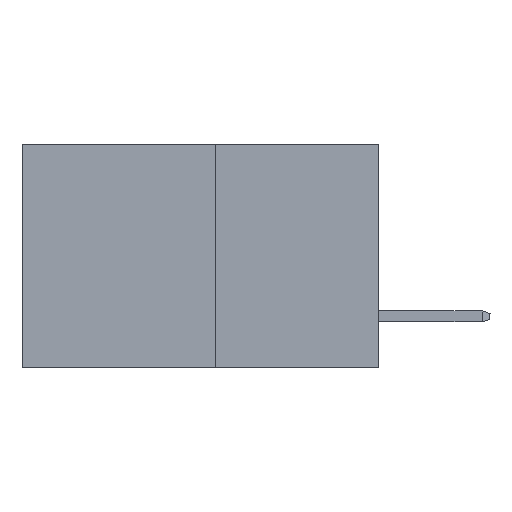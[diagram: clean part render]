
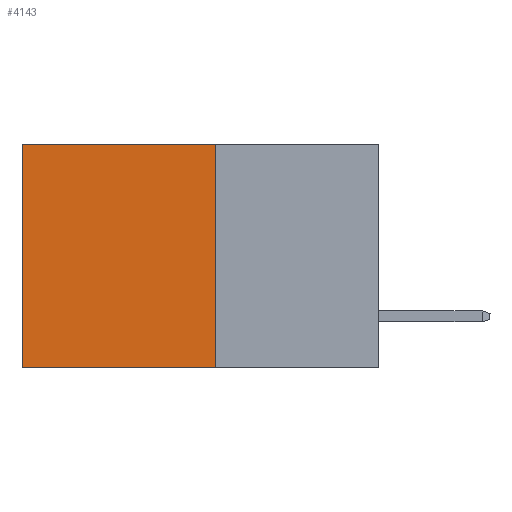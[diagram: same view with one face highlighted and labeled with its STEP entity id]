
A CAD part, left-side view. The second image highlights one B-rep face of the part: STEP entity #4143.
In plain terms, the highlighted planar face has unit normal (-1, 0, 0).
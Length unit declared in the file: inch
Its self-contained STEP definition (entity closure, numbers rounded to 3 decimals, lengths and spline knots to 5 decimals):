
#330 = VERTEX_POINT ( 'NONE', #10010 ) ;
#670 = VERTEX_POINT ( 'NONE', #10265 ) ;
#835 = CARTESIAN_POINT ( 'NONE',  ( 0.277, 0.27, -0.37 ) ) ;
#922 = EDGE_CURVE ( 'NONE', #2797, #670, #10425, .T. ) ;
#929 = ORIENTED_EDGE ( 'NONE', *, *, #11727, .T. ) ;
#1316 = FACE_OUTER_BOUND ( 'NONE', #10411, .T. ) ;
#1929 = EDGE_CURVE ( 'NONE', #330, #2797, #5832, .T. ) ;
#2237 = VECTOR ( 'NONE', #5999, 39.37008 ) ;
#2704 = CARTESIAN_POINT ( 'NONE',  ( 0.277, 0.27, -0.37 ) ) ;
#2732 = DIRECTION ( 'NONE',  ( 0., 1., 0. ) ) ;
#2797 = VERTEX_POINT ( 'NONE', #5169 ) ;
#3555 = VECTOR ( 'NONE', #8559, 39.37008 ) ;
#3775 = ORIENTED_EDGE ( 'NONE', *, *, #1929, .F. ) ;
#3859 = PLANE ( 'NONE',  #8835 ) ;
#4143 = ADVANCED_FACE ( 'NONE', ( #1316 ), #3859, .F. ) ;
#4469 = CARTESIAN_POINT ( 'NONE',  ( 0.277, 0.59, 0. ) ) ;
#5169 = CARTESIAN_POINT ( 'NONE',  ( 0.277, 0.27, -0.37 ) ) ;
#5832 = LINE ( 'NONE', #835, #3555 ) ;
#5999 = DIRECTION ( 'NONE',  ( 0., 0., -1. ) ) ;
#6320 = ORIENTED_EDGE ( 'NONE', *, *, #922, .F. ) ;
#6413 = LINE ( 'NONE', #9970, #9027 ) ;
#6484 = DIRECTION ( 'NONE',  ( 1., 0., 0. ) ) ;
#7861 = VECTOR ( 'NONE', #11091, 39.37008 ) ;
#8559 = DIRECTION ( 'NONE',  ( 0., 0., -1. ) ) ;
#8835 = AXIS2_PLACEMENT_3D ( 'NONE', #13249, #6484, #11849 ) ;
#8981 = VERTEX_POINT ( 'NONE', #4469 ) ;
#9027 = VECTOR ( 'NONE', #2732, 39.37008 ) ;
#9970 = CARTESIAN_POINT ( 'NONE',  ( 0.277, 0.27, 0. ) ) ;
#10010 = CARTESIAN_POINT ( 'NONE',  ( 0.277, 0.27, 0. ) ) ;
#10265 = CARTESIAN_POINT ( 'NONE',  ( 0.277, 0.59, -0.37 ) ) ;
#10411 = EDGE_LOOP ( 'NONE', ( #13277, #6320, #3775, #929 ) ) ;
#10425 = LINE ( 'NONE', #2704, #7861 ) ;
#10518 = LINE ( 'NONE', #10801, #2237 ) ;
#10635 = EDGE_CURVE ( 'NONE', #8981, #670, #10518, .T. ) ;
#10801 = CARTESIAN_POINT ( 'NONE',  ( 0.277, 0.59, -0.37 ) ) ;
#11091 = DIRECTION ( 'NONE',  ( 0., 1., 0. ) ) ;
#11727 = EDGE_CURVE ( 'NONE', #330, #8981, #6413, .T. ) ;
#11849 = DIRECTION ( 'NONE',  ( 0., 0., -1. ) ) ;
#13249 = CARTESIAN_POINT ( 'NONE',  ( 0.277, 0.27, -0.37 ) ) ;
#13277 = ORIENTED_EDGE ( 'NONE', *, *, #10635, .T. ) ;
